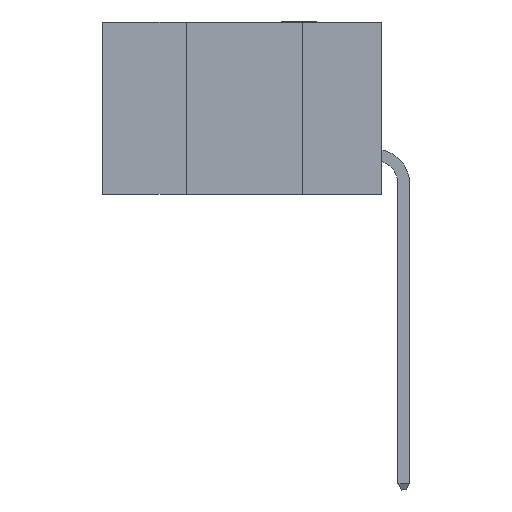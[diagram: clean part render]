
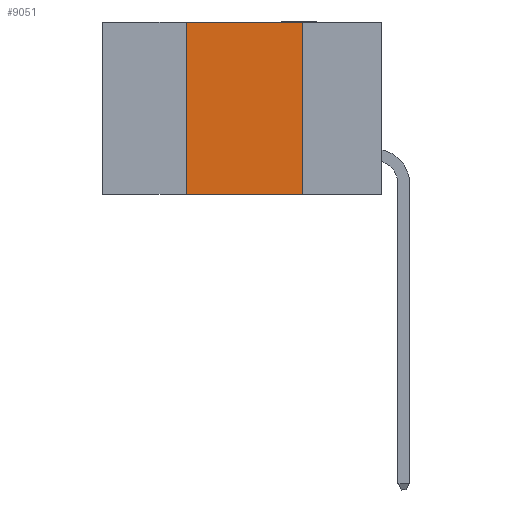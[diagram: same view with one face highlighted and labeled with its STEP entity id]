
A CAD part, left-side view. The second image highlights one B-rep face of the part: STEP entity #9051.
In plain terms, the highlighted planar face has unit normal (-1, 0, 0).
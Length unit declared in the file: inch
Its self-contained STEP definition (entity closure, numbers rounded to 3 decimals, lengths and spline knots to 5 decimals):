
#40 = VECTOR ( 'NONE', #11956, 39.37008 ) ;
#107 = CARTESIAN_POINT ( 'NONE',  ( 0., 0.6, 0. ) ) ;
#218 = EDGE_CURVE ( 'NONE', #9721, #9973, #11619, .T. ) ;
#1471 = DIRECTION ( 'NONE',  ( 1., 0., 0. ) ) ;
#2599 = LINE ( 'NONE', #14244, #5694 ) ;
#2936 = EDGE_CURVE ( 'NONE', #10838, #8970, #7038, .T. ) ;
#3450 = AXIS2_PLACEMENT_3D ( 'NONE', #107, #1471, #10432 ) ;
#3983 = CARTESIAN_POINT ( 'NONE',  ( 0., 0.17, 0. ) ) ;
#4131 = CARTESIAN_POINT ( 'NONE',  ( 0., 0.42, -0.37 ) ) ;
#4763 = CARTESIAN_POINT ( 'NONE',  ( 0., 0.42, 0. ) ) ;
#5302 = DIRECTION ( 'NONE',  ( 0., 0., 1. ) ) ;
#5378 = ORIENTED_EDGE ( 'NONE', *, *, #7916, .F. ) ;
#5511 = EDGE_LOOP ( 'NONE', ( #15339, #5378, #14369, #5653 ) ) ;
#5653 = ORIENTED_EDGE ( 'NONE', *, *, #10241, .T. ) ;
#5694 = VECTOR ( 'NONE', #8122, 39.37008 ) ;
#6432 = CARTESIAN_POINT ( 'NONE',  ( 0., 0.17, -0.37 ) ) ;
#7038 = LINE ( 'NONE', #15435, #40 ) ;
#7755 = DIRECTION ( 'NONE',  ( 0., -1., 0. ) ) ;
#7916 = EDGE_CURVE ( 'NONE', #9973, #10838, #2599, .T. ) ;
#8122 = DIRECTION ( 'NONE',  ( 0., -1., 0. ) ) ;
#8970 = VERTEX_POINT ( 'NONE', #6432 ) ;
#9051 = ADVANCED_FACE ( 'NONE', ( #14526 ), #14095, .F. ) ;
#9373 = LINE ( 'NONE', #16322, #15852 ) ;
#9721 = VERTEX_POINT ( 'NONE', #4131 ) ;
#9973 = VERTEX_POINT ( 'NONE', #10891 ) ;
#10241 = EDGE_CURVE ( 'NONE', #9721, #8970, #9373, .T. ) ;
#10432 = DIRECTION ( 'NONE',  ( 0., 0., -1. ) ) ;
#10838 = VERTEX_POINT ( 'NONE', #3983 ) ;
#10891 = CARTESIAN_POINT ( 'NONE',  ( 0., 0.42, 0. ) ) ;
#11197 = VECTOR ( 'NONE', #5302, 39.37008 ) ;
#11619 = LINE ( 'NONE', #4763, #11197 ) ;
#11956 = DIRECTION ( 'NONE',  ( 0., 0., -1. ) ) ;
#14095 = PLANE ( 'NONE',  #3450 ) ;
#14244 = CARTESIAN_POINT ( 'NONE',  ( 0., 0.6, 0. ) ) ;
#14369 = ORIENTED_EDGE ( 'NONE', *, *, #218, .F. ) ;
#14526 = FACE_OUTER_BOUND ( 'NONE', #5511, .T. ) ;
#15339 = ORIENTED_EDGE ( 'NONE', *, *, #2936, .F. ) ;
#15435 = CARTESIAN_POINT ( 'NONE',  ( 0., 0.17, 0. ) ) ;
#15852 = VECTOR ( 'NONE', #7755, 39.37008 ) ;
#16322 = CARTESIAN_POINT ( 'NONE',  ( 0., 0.6, -0.37 ) ) ;
